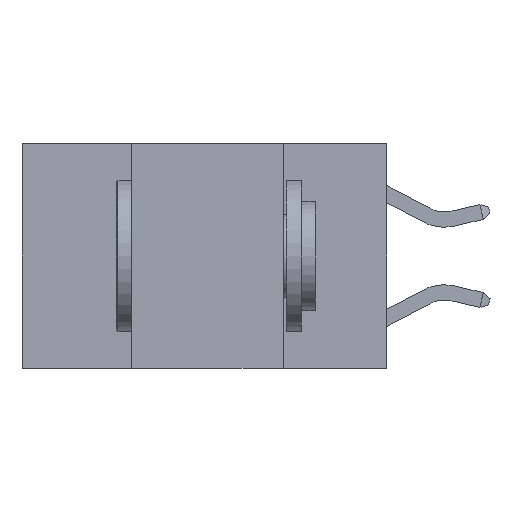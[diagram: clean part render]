
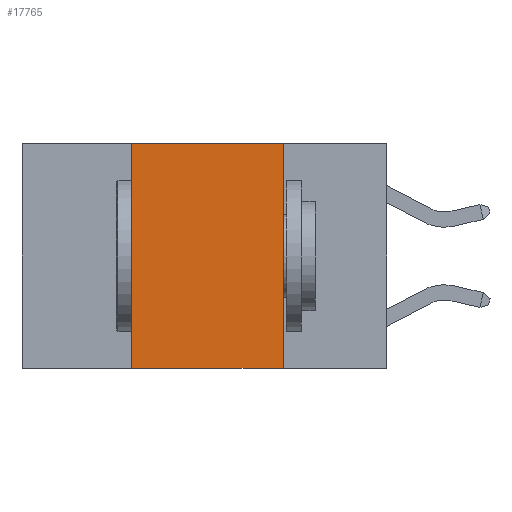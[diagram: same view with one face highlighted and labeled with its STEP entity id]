
A CAD part, left-side view. The second image highlights one B-rep face of the part: STEP entity #17765.
In plain terms, the highlighted planar face has unit normal (-1, 0, 0).
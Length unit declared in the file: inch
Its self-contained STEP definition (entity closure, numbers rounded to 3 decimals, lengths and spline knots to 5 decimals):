
#537 = DIRECTION ( 'NONE',  ( 0., 0., -1. ) ) ;
#652 = CARTESIAN_POINT ( 'NONE',  ( 0., 0.6, 0. ) ) ;
#705 = DIRECTION ( 'NONE',  ( 0., 0., 1. ) ) ;
#710 = AXIS2_PLACEMENT_3D ( 'NONE', #15582, #21938, #17816 ) ;
#1105 = LINE ( 'NONE', #24071, #16987 ) ;
#3009 = DIRECTION ( 'NONE',  ( 0., -1., 0. ) ) ;
#4506 = EDGE_CURVE ( 'NONE', #6032, #21906, #15892, .T. ) ;
#4671 = LINE ( 'NONE', #9230, #13937 ) ;
#6032 = VERTEX_POINT ( 'NONE', #8532 ) ;
#8532 = CARTESIAN_POINT ( 'NONE',  ( 0., 0.42, 0. ) ) ;
#9230 = CARTESIAN_POINT ( 'NONE',  ( 0., 0.17, 0. ) ) ;
#9456 = FACE_OUTER_BOUND ( 'NONE', #24912, .T. ) ;
#9554 = VECTOR ( 'NONE', #705, 39.37008 ) ;
#10861 = VERTEX_POINT ( 'NONE', #12060 ) ;
#11073 = LINE ( 'NONE', #19550, #9554 ) ;
#12013 = ORIENTED_EDGE ( 'NONE', *, *, #20104, .T. ) ;
#12060 = CARTESIAN_POINT ( 'NONE',  ( 0., 0.17, -0.37 ) ) ;
#12492 = ORIENTED_EDGE ( 'NONE', *, *, #22803, .F. ) ;
#13561 = DIRECTION ( 'NONE',  ( 0., -1., 0. ) ) ;
#13937 = VECTOR ( 'NONE', #537, 39.37008 ) ;
#15582 = CARTESIAN_POINT ( 'NONE',  ( 0., 0.6, 0. ) ) ;
#15892 = LINE ( 'NONE', #652, #17124 ) ;
#16868 = ORIENTED_EDGE ( 'NONE', *, *, #23651, .F. ) ;
#16987 = VECTOR ( 'NONE', #13561, 39.37008 ) ;
#17124 = VECTOR ( 'NONE', #3009, 39.37008 ) ;
#17765 = ADVANCED_FACE ( 'NONE', ( #9456 ), #26496, .F. ) ;
#17816 = DIRECTION ( 'NONE',  ( 0., 0., -1. ) ) ;
#18276 = ORIENTED_EDGE ( 'NONE', *, *, #4506, .F. ) ;
#19550 = CARTESIAN_POINT ( 'NONE',  ( 0., 0.42, 0. ) ) ;
#20044 = CARTESIAN_POINT ( 'NONE',  ( 0., 0.17, 0. ) ) ;
#20104 = EDGE_CURVE ( 'NONE', #26727, #10861, #1105, .T. ) ;
#21906 = VERTEX_POINT ( 'NONE', #20044 ) ;
#21938 = DIRECTION ( 'NONE',  ( 1., 0., 0. ) ) ;
#22568 = CARTESIAN_POINT ( 'NONE',  ( 0., 0.42, -0.37 ) ) ;
#22803 = EDGE_CURVE ( 'NONE', #21906, #10861, #4671, .T. ) ;
#23651 = EDGE_CURVE ( 'NONE', #26727, #6032, #11073, .T. ) ;
#24071 = CARTESIAN_POINT ( 'NONE',  ( 0., 0.6, -0.37 ) ) ;
#24912 = EDGE_LOOP ( 'NONE', ( #12492, #18276, #16868, #12013 ) ) ;
#26496 = PLANE ( 'NONE',  #710 ) ;
#26727 = VERTEX_POINT ( 'NONE', #22568 ) ;
